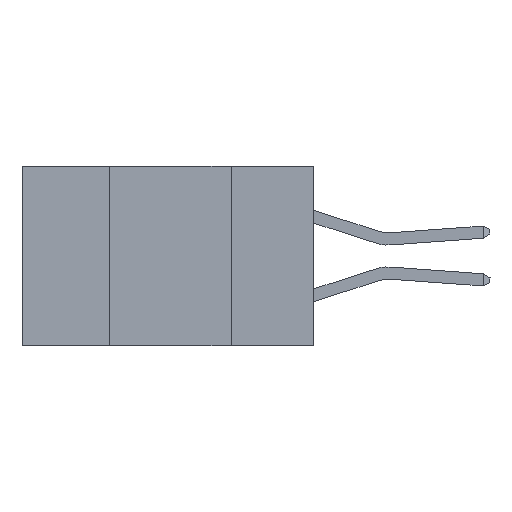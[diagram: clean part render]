
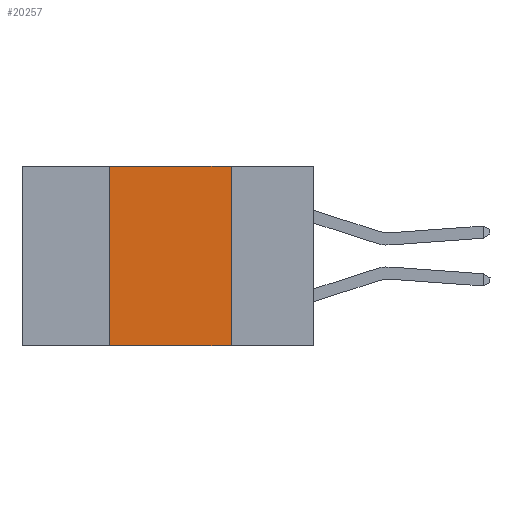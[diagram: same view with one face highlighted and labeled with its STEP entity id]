
A CAD part, left-side view. The second image highlights one B-rep face of the part: STEP entity #20257.
In plain terms, the highlighted planar face has unit normal (-1, 0, 0).
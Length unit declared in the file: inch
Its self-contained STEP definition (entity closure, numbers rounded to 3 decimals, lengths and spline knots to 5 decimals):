
#33 = EDGE_CURVE ( 'NONE', #15604, #6002, #5960, .T. ) ;
#493 = CARTESIAN_POINT ( 'NONE',  ( 0., 0.6, 0. ) ) ;
#563 = AXIS2_PLACEMENT_3D ( 'NONE', #12185, #14594, #14453 ) ;
#631 = EDGE_CURVE ( 'NONE', #9366, #18605, #10597, .T. ) ;
#1577 = CARTESIAN_POINT ( 'NONE',  ( 0., 0.17, 0. ) ) ;
#1996 = VECTOR ( 'NONE', #24575, 39.37008 ) ;
#3297 = FACE_OUTER_BOUND ( 'NONE', #6560, .T. ) ;
#3919 = ORIENTED_EDGE ( 'NONE', *, *, #631, .F. ) ;
#4527 = LINE ( 'NONE', #18687, #14183 ) ;
#5452 = LINE ( 'NONE', #493, #25054 ) ;
#5580 = EDGE_CURVE ( 'NONE', #15604, #18605, #4527, .T. ) ;
#5960 = LINE ( 'NONE', #8088, #18179 ) ;
#6002 = VERTEX_POINT ( 'NONE', #11572 ) ;
#6560 = EDGE_LOOP ( 'NONE', ( #3919, #10808, #10706, #19390 ) ) ;
#8088 = CARTESIAN_POINT ( 'NONE',  ( 0., 0.42, 0. ) ) ;
#9366 = VERTEX_POINT ( 'NONE', #1577 ) ;
#9638 = DIRECTION ( 'NONE',  ( 0., -1., 0. ) ) ;
#9946 = CARTESIAN_POINT ( 'NONE',  ( 0., 0.17, -0.37 ) ) ;
#10043 = DIRECTION ( 'NONE',  ( 0., 0., 1. ) ) ;
#10597 = LINE ( 'NONE', #22769, #1996 ) ;
#10706 = ORIENTED_EDGE ( 'NONE', *, *, #33, .F. ) ;
#10808 = ORIENTED_EDGE ( 'NONE', *, *, #18127, .F. ) ;
#11572 = CARTESIAN_POINT ( 'NONE',  ( 0., 0.42, 0. ) ) ;
#12185 = CARTESIAN_POINT ( 'NONE',  ( 0., 0.6, 0. ) ) ;
#14183 = VECTOR ( 'NONE', #9638, 39.37008 ) ;
#14453 = DIRECTION ( 'NONE',  ( 0., 0., -1. ) ) ;
#14594 = DIRECTION ( 'NONE',  ( 1., 0., 0. ) ) ;
#15604 = VERTEX_POINT ( 'NONE', #28319 ) ;
#16720 = PLANE ( 'NONE',  #563 ) ;
#18127 = EDGE_CURVE ( 'NONE', #6002, #9366, #5452, .T. ) ;
#18179 = VECTOR ( 'NONE', #10043, 39.37008 ) ;
#18605 = VERTEX_POINT ( 'NONE', #9946 ) ;
#18687 = CARTESIAN_POINT ( 'NONE',  ( 0., 0.6, -0.37 ) ) ;
#19390 = ORIENTED_EDGE ( 'NONE', *, *, #5580, .T. ) ;
#20257 = ADVANCED_FACE ( 'NONE', ( #3297 ), #16720, .F. ) ;
#22769 = CARTESIAN_POINT ( 'NONE',  ( 0., 0.17, 0. ) ) ;
#24575 = DIRECTION ( 'NONE',  ( 0., 0., -1. ) ) ;
#25054 = VECTOR ( 'NONE', #28178, 39.37008 ) ;
#28178 = DIRECTION ( 'NONE',  ( 0., -1., 0. ) ) ;
#28319 = CARTESIAN_POINT ( 'NONE',  ( 0., 0.42, -0.37 ) ) ;
